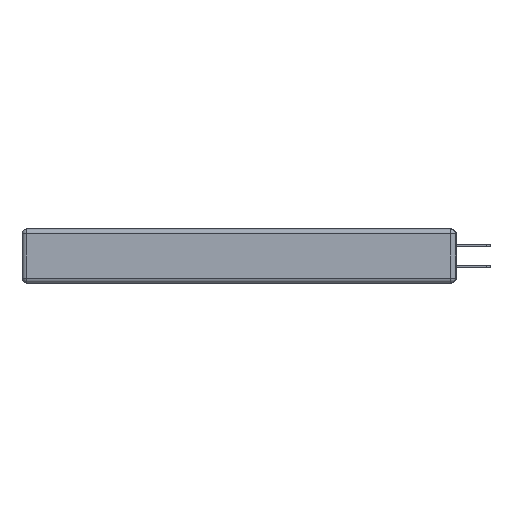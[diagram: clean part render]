
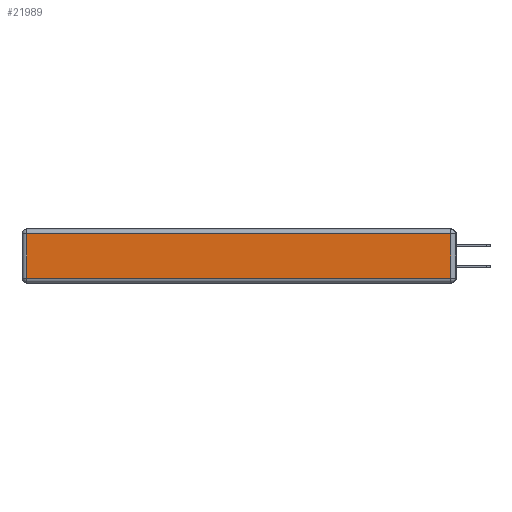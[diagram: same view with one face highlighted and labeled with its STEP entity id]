
A CAD part, left-side view. The second image highlights one B-rep face of the part: STEP entity #21989.
In plain terms, the highlighted planar face has unit normal (-1, 0, 0).
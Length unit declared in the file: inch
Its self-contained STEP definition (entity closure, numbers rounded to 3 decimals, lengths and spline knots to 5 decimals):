
#837 = ORIENTED_EDGE ( 'NONE', *, *, #13248, .T. ) ;
#1215 = DIRECTION ( 'NONE',  ( 0., -1., 0. ) ) ;
#1479 = CARTESIAN_POINT ( 'NONE',  ( 0., 0.03, -0.03 ) ) ;
#1592 = FACE_OUTER_BOUND ( 'NONE', #16159, .T. ) ;
#2394 = VECTOR ( 'NONE', #21761, 39.37008 ) ;
#2674 = LINE ( 'NONE', #8966, #2394 ) ;
#2830 = CARTESIAN_POINT ( 'NONE',  ( 0., 0., -0.313 ) ) ;
#3980 = EDGE_CURVE ( 'NONE', #23060, #23135, #14808, .T. ) ;
#4686 = DIRECTION ( 'NONE',  ( 0., 0., 1. ) ) ;
#4759 = AXIS2_PLACEMENT_3D ( 'NONE', #18490, #9310, #21997 ) ;
#5204 = ORIENTED_EDGE ( 'NONE', *, *, #22178, .T. ) ;
#7314 = LINE ( 'NONE', #13665, #20982 ) ;
#8099 = VERTEX_POINT ( 'NONE', #22841 ) ;
#8172 = ORIENTED_EDGE ( 'NONE', *, *, #3980, .T. ) ;
#8966 = CARTESIAN_POINT ( 'NONE',  ( 0., 2.72, -0.343 ) ) ;
#9310 = DIRECTION ( 'NONE',  ( -1., 0., 0. ) ) ;
#10485 = CARTESIAN_POINT ( 'NONE',  ( 0., 0.03, -0.343 ) ) ;
#12875 = EDGE_CURVE ( 'NONE', #8099, #23060, #2674, .T. ) ;
#13248 = EDGE_CURVE ( 'NONE', #14946, #8099, #7314, .T. ) ;
#13665 = CARTESIAN_POINT ( 'NONE',  ( 0., 2.75, -0.03 ) ) ;
#14808 = LINE ( 'NONE', #2830, #20339 ) ;
#14946 = VERTEX_POINT ( 'NONE', #1479 ) ;
#15129 = VECTOR ( 'NONE', #4686, 39.37008 ) ;
#16159 = EDGE_LOOP ( 'NONE', ( #8172, #5204, #837, #18751 ) ) ;
#18490 = CARTESIAN_POINT ( 'NONE',  ( 0., 0., -0.343 ) ) ;
#18751 = ORIENTED_EDGE ( 'NONE', *, *, #12875, .T. ) ;
#19259 = DIRECTION ( 'NONE',  ( 0., 1., 0. ) ) ;
#20339 = VECTOR ( 'NONE', #1215, 39.37008 ) ;
#20418 = CARTESIAN_POINT ( 'NONE',  ( 0., 2.72, -0.313 ) ) ;
#20982 = VECTOR ( 'NONE', #19259, 39.37008 ) ;
#21761 = DIRECTION ( 'NONE',  ( 0., 0., -1. ) ) ;
#21989 = ADVANCED_FACE ( 'NONE', ( #1592 ), #22328, .T. ) ;
#21997 = DIRECTION ( 'NONE',  ( 0., 0., 1. ) ) ;
#22178 = EDGE_CURVE ( 'NONE', #23135, #14946, #23280, .T. ) ;
#22328 = PLANE ( 'NONE',  #4759 ) ;
#22841 = CARTESIAN_POINT ( 'NONE',  ( 0., 2.72, -0.03 ) ) ;
#23005 = CARTESIAN_POINT ( 'NONE',  ( 0., 0.03, -0.313 ) ) ;
#23060 = VERTEX_POINT ( 'NONE', #20418 ) ;
#23135 = VERTEX_POINT ( 'NONE', #23005 ) ;
#23280 = LINE ( 'NONE', #10485, #15129 ) ;
